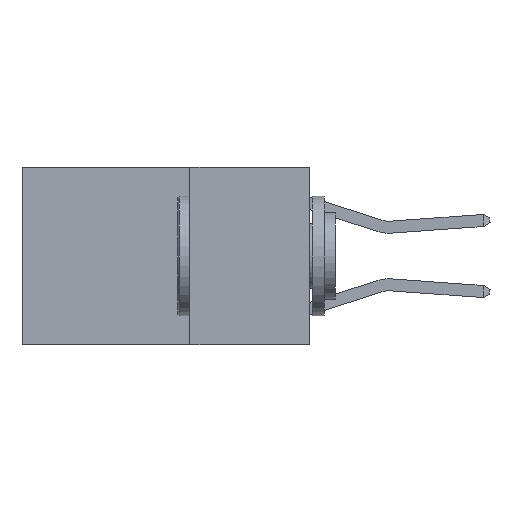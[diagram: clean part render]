
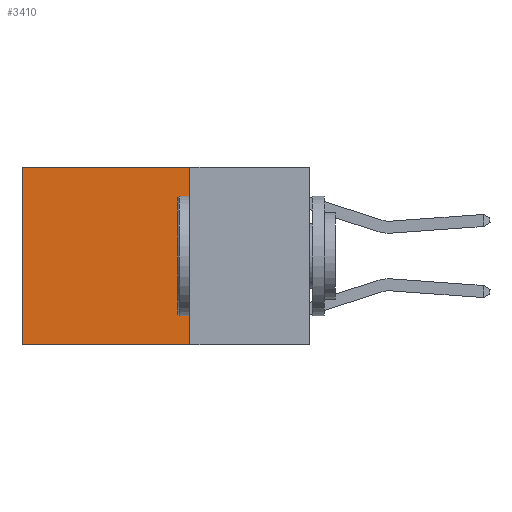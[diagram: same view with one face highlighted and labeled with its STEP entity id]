
A CAD part, left-side view. The second image highlights one B-rep face of the part: STEP entity #3410.
In plain terms, the highlighted planar face has unit normal (-1, 0, 0).
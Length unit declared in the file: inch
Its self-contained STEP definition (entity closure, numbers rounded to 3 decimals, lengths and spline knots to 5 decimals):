
#224 = DIRECTION ( 'NONE',  ( 0., 0., -1. ) ) ;
#507 = VECTOR ( 'NONE', #9277, 39.37008 ) ;
#766 = VERTEX_POINT ( 'NONE', #3363 ) ;
#838 = ORIENTED_EDGE ( 'NONE', *, *, #8524, .F. ) ;
#1086 = PLANE ( 'NONE',  #12384 ) ;
#1449 = LINE ( 'NONE', #4521, #9382 ) ;
#2152 = DIRECTION ( 'NONE',  ( 1., 0., 0. ) ) ;
#2917 = VERTEX_POINT ( 'NONE', #6014 ) ;
#3363 = CARTESIAN_POINT ( 'NONE',  ( 0.2625, 0.25, 0. ) ) ;
#3410 = ADVANCED_FACE ( 'NONE', ( #10136 ), #1086, .F. ) ;
#4521 = CARTESIAN_POINT ( 'NONE',  ( 0.2625, 0.25, -0.37 ) ) ;
#5173 = CARTESIAN_POINT ( 'NONE',  ( 0.2625, 0.25, 0. ) ) ;
#5950 = EDGE_CURVE ( 'NONE', #2917, #7623, #6291, .T. ) ;
#6006 = CARTESIAN_POINT ( 'NONE',  ( 0.2625, 0.6, -0.37 ) ) ;
#6014 = CARTESIAN_POINT ( 'NONE',  ( 0.2625, 0.6, 0. ) ) ;
#6291 = LINE ( 'NONE', #10258, #507 ) ;
#7071 = EDGE_LOOP ( 'NONE', ( #11405, #838, #8855, #8418 ) ) ;
#7262 = VERTEX_POINT ( 'NONE', #8594 ) ;
#7623 = VERTEX_POINT ( 'NONE', #6006 ) ;
#8418 = ORIENTED_EDGE ( 'NONE', *, *, #8941, .T. ) ;
#8524 = EDGE_CURVE ( 'NONE', #7262, #7623, #1449, .T. ) ;
#8594 = CARTESIAN_POINT ( 'NONE',  ( 0.2625, 0.25, -0.37 ) ) ;
#8645 = LINE ( 'NONE', #12572, #10011 ) ;
#8845 = VECTOR ( 'NONE', #224, 39.37008 ) ;
#8855 = ORIENTED_EDGE ( 'NONE', *, *, #11907, .F. ) ;
#8941 = EDGE_CURVE ( 'NONE', #766, #2917, #8645, .T. ) ;
#9170 = DIRECTION ( 'NONE',  ( 0., 0., -1. ) ) ;
#9277 = DIRECTION ( 'NONE',  ( 0., 0., -1. ) ) ;
#9290 = CARTESIAN_POINT ( 'NONE',  ( 0.2625, 0.25, 0. ) ) ;
#9382 = VECTOR ( 'NONE', #12308, 39.37008 ) ;
#10011 = VECTOR ( 'NONE', #10456, 39.37008 ) ;
#10136 = FACE_OUTER_BOUND ( 'NONE', #7071, .T. ) ;
#10258 = CARTESIAN_POINT ( 'NONE',  ( 0.2625, 0.6, 0. ) ) ;
#10456 = DIRECTION ( 'NONE',  ( 0., 1., 0. ) ) ;
#11405 = ORIENTED_EDGE ( 'NONE', *, *, #5950, .T. ) ;
#11907 = EDGE_CURVE ( 'NONE', #766, #7262, #12256, .T. ) ;
#12256 = LINE ( 'NONE', #9290, #8845 ) ;
#12308 = DIRECTION ( 'NONE',  ( 0., 1., 0. ) ) ;
#12384 = AXIS2_PLACEMENT_3D ( 'NONE', #5173, #2152, #9170 ) ;
#12572 = CARTESIAN_POINT ( 'NONE',  ( 0.2625, 0.25, 0. ) ) ;
